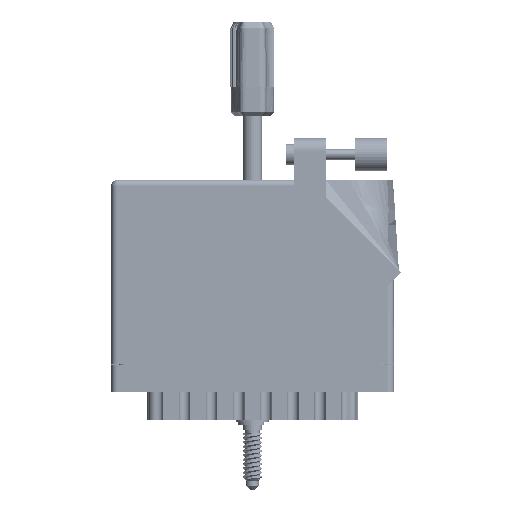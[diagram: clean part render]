
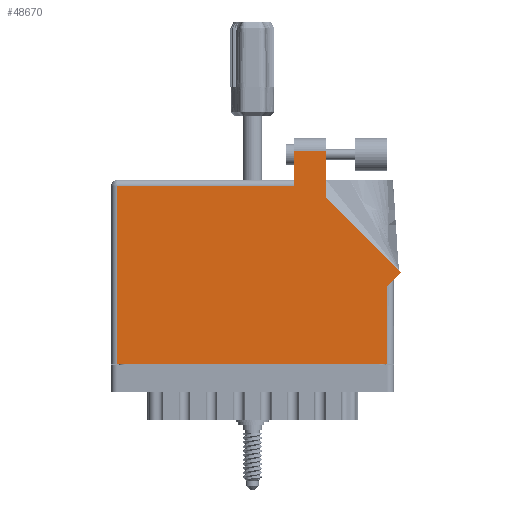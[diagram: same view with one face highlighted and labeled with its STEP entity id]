
A CAD part, front view. The second image highlights one B-rep face of the part: STEP entity #48670.
In plain terms, the highlighted face is planar.
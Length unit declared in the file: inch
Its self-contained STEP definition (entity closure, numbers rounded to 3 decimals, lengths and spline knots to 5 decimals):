
#1158 = VECTOR ( 'NONE', #40632, 39.37008 ) ;
#1405 = EDGE_CURVE ( 'NONE', #30309, #45439, #44063, .T. ) ;
#2519 = VERTEX_POINT ( 'NONE', #42877 ) ;
#4952 = VERTEX_POINT ( 'NONE', #54306 ) ;
#5192 = EDGE_CURVE ( 'NONE', #4952, #50850, #8132, .T. ) ;
#6809 = DIRECTION ( 'NONE',  ( -1., 0., 0. ) ) ;
#6868 = EDGE_CURVE ( 'NONE', #27995, #4952, #41279, .T. ) ;
#8132 = LINE ( 'NONE', #8649, #79454 ) ;
#8376 = VERTEX_POINT ( 'NONE', #79341 ) ;
#8649 = CARTESIAN_POINT ( 'NONE',  ( 2.065, 1.60942, 0. ) ) ;
#8822 = PLANE ( 'NONE',  #80564 ) ;
#9435 = VERTEX_POINT ( 'NONE', #49821 ) ;
#10491 = ORIENTED_EDGE ( 'NONE', *, *, #72002, .T. ) ;
#11005 = VECTOR ( 'NONE', #74195, 39.37008 ) ;
#11194 = ORIENTED_EDGE ( 'NONE', *, *, #69748, .T. ) ;
#13129 = CARTESIAN_POINT ( 'NONE',  ( 0.062, 1.713, 0. ) ) ;
#14073 = EDGE_CURVE ( 'NONE', #8376, #27995, #47138, .T. ) ;
#15454 = DIRECTION ( 'NONE',  ( 0., 0., -1. ) ) ;
#16046 = CARTESIAN_POINT ( 'NONE',  ( 0., 1.775, 0. ) ) ;
#16599 = DIRECTION ( 'NONE',  ( 0., 1., 0. ) ) ;
#20351 = ORIENTED_EDGE ( 'NONE', *, *, #14073, .T. ) ;
#21123 = CARTESIAN_POINT ( 'NONE',  ( 0.062, 0., 0. ) ) ;
#23179 = ORIENTED_EDGE ( 'NONE', *, *, #5192, .T. ) ;
#24036 = ORIENTED_EDGE ( 'NONE', *, *, #1405, .T. ) ;
#25590 = VECTOR ( 'NONE', #80968, 39.37008 ) ;
#27767 = ORIENTED_EDGE ( 'NONE', *, *, #6868, .T. ) ;
#27995 = VERTEX_POINT ( 'NONE', #62356 ) ;
#29462 = DIRECTION ( 'NONE',  ( 0., 1., 0. ) ) ;
#30277 = DIRECTION ( 'NONE',  ( 0., -1., 0. ) ) ;
#30309 = VERTEX_POINT ( 'NONE', #52402 ) ;
#31429 = LINE ( 'NONE', #46687, #1158 ) ;
#32812 = CARTESIAN_POINT ( 'NONE',  ( 0., 1.713, 0. ) ) ;
#33489 = VERTEX_POINT ( 'NONE', #81176 ) ;
#34638 = ORIENTED_EDGE ( 'NONE', *, *, #81524, .T. ) ;
#35406 = LINE ( 'NONE', #36875, #53799 ) ;
#36875 = CARTESIAN_POINT ( 'NONE',  ( 1.758, 1.775, 0. ) ) ;
#38106 = LINE ( 'NONE', #57786, #81351 ) ;
#40632 = DIRECTION ( 'NONE',  ( 1., 0., 0. ) ) ;
#41279 = LINE ( 'NONE', #55448, #11005 ) ;
#42877 = CARTESIAN_POINT ( 'NONE',  ( 1.758, 2.05, 0. ) ) ;
#43628 = VECTOR ( 'NONE', #6809, 39.37008 ) ;
#44063 = LINE ( 'NONE', #32812, #79758 ) ;
#45439 = VERTEX_POINT ( 'NONE', #13129 ) ;
#45826 = LINE ( 'NONE', #60582, #43628 ) ;
#46687 = CARTESIAN_POINT ( 'NONE',  ( 0., 0., 0. ) ) ;
#47138 = LINE ( 'NONE', #87582, #25590 ) ;
#47452 = CARTESIAN_POINT ( 'NONE',  ( 2.065, 2.05, 0. ) ) ;
#48670 = ADVANCED_FACE ( 'NONE', ( #56601 ), #8822, .F. ) ;
#49821 = CARTESIAN_POINT ( 'NONE',  ( 2.656, 0., 0. ) ) ;
#50850 = VERTEX_POINT ( 'NONE', #47452 ) ;
#52377 = EDGE_CURVE ( 'NONE', #33489, #9435, #31429, .T. ) ;
#52402 = CARTESIAN_POINT ( 'NONE',  ( 1.758, 1.713, 0. ) ) ;
#52864 = ORIENTED_EDGE ( 'NONE', *, *, #87769, .T. ) ;
#53799 = VECTOR ( 'NONE', #30277, 39.37008 ) ;
#54306 = CARTESIAN_POINT ( 'NONE',  ( 2.065, 1.60942, 0. ) ) ;
#55448 = CARTESIAN_POINT ( 'NONE',  ( 2.78871, 0.88571, 0. ) ) ;
#56601 = FACE_OUTER_BOUND ( 'NONE', #62727, .T. ) ;
#57786 = CARTESIAN_POINT ( 'NONE',  ( 2.656, 0.815, 0. ) ) ;
#60048 = VECTOR ( 'NONE', #89400, 39.37008 ) ;
#60582 = CARTESIAN_POINT ( 'NONE',  ( 1.758, 2.05, 0. ) ) ;
#60858 = DIRECTION ( 'NONE',  ( -1., 0., 0. ) ) ;
#62356 = CARTESIAN_POINT ( 'NONE',  ( 2.78871, 0.88571, 0. ) ) ;
#62727 = EDGE_LOOP ( 'NONE', ( #23179, #52864, #11194, #24036, #10491, #68232, #34638, #20351, #27767 ) ) ;
#68232 = ORIENTED_EDGE ( 'NONE', *, *, #52377, .T. ) ;
#69748 = EDGE_CURVE ( 'NONE', #2519, #30309, #35406, .T. ) ;
#71905 = LINE ( 'NONE', #21123, #60048 ) ;
#72002 = EDGE_CURVE ( 'NONE', #45439, #33489, #71905, .T. ) ;
#74195 = DIRECTION ( 'NONE',  ( -0.707, 0.707, 0. ) ) ;
#77946 = DIRECTION ( 'NONE',  ( -1., 0., 0. ) ) ;
#79341 = CARTESIAN_POINT ( 'NONE',  ( 2.656, 0.753, 0. ) ) ;
#79454 = VECTOR ( 'NONE', #16599, 39.37008 ) ;
#79758 = VECTOR ( 'NONE', #60858, 39.37008 ) ;
#80564 = AXIS2_PLACEMENT_3D ( 'NONE', #16046, #15454, #77946 ) ;
#80968 = DIRECTION ( 'NONE',  ( 0.707, 0.707, 0. ) ) ;
#81176 = CARTESIAN_POINT ( 'NONE',  ( 0.062, 0., 0. ) ) ;
#81351 = VECTOR ( 'NONE', #29462, 39.37008 ) ;
#81524 = EDGE_CURVE ( 'NONE', #9435, #8376, #38106, .T. ) ;
#87582 = CARTESIAN_POINT ( 'NONE',  ( 2.718, 0.815, 0. ) ) ;
#87769 = EDGE_CURVE ( 'NONE', #50850, #2519, #45826, .T. ) ;
#89400 = DIRECTION ( 'NONE',  ( 0., -1., 0. ) ) ;
